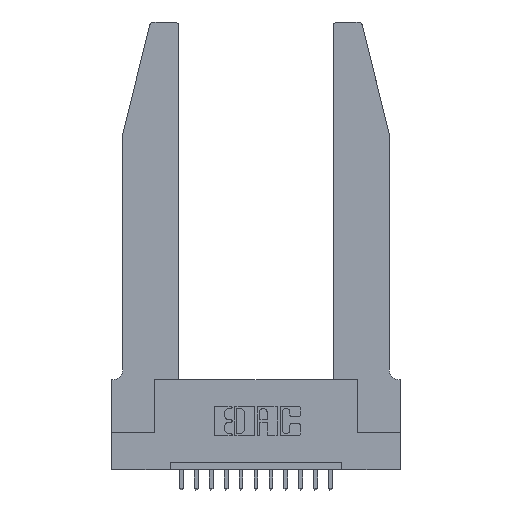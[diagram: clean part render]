
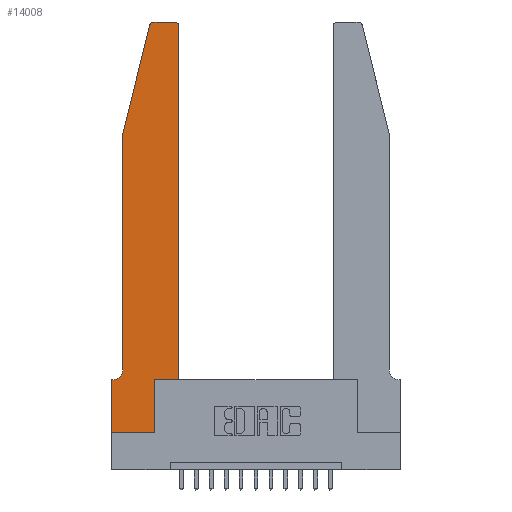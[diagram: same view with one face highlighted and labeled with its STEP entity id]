
A CAD part, top view. The second image highlights one B-rep face of the part: STEP entity #14008.
In plain terms, the highlighted planar face has unit normal (0, 0, 1).
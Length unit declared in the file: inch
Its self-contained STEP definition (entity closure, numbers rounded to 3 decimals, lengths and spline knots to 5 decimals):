
#631 = CARTESIAN_POINT ( 'NONE',  ( 0.284, 2.72, 0.37 ) ) ;
#816 = VECTOR ( 'NONE', #4452, 39.37008 ) ;
#818 = DIRECTION ( 'NONE',  ( -1., 0., 0. ) ) ;
#859 = CARTESIAN_POINT ( 'NONE',  ( 0.4205, 2.72, 0.37 ) ) ;
#905 = CARTESIAN_POINT ( 'NONE',  ( 0.0755, 2., 0.37 ) ) ;
#1058 = VERTEX_POINT ( 'NONE', #8115 ) ;
#1556 = CARTESIAN_POINT ( 'NONE',  ( 0., 0., 0.37 ) ) ;
#1710 = DIRECTION ( 'NONE',  ( 0., 1., 0. ) ) ;
#2097 = DIRECTION ( 'NONE',  ( 1., 0., 0. ) ) ;
#2115 = ORIENTED_EDGE ( 'NONE', *, *, #4178, .T. ) ;
#2126 = VERTEX_POINT ( 'NONE', #14077 ) ;
#2444 = VECTOR ( 'NONE', #7209, 39.37008 ) ;
#2479 = CARTESIAN_POINT ( 'NONE',  ( 0.0755, 2., 0.37 ) ) ;
#2604 = AXIS2_PLACEMENT_3D ( 'NONE', #859, #3654, #2097 ) ;
#2664 = ORIENTED_EDGE ( 'NONE', *, *, #14502, .T. ) ;
#2697 = DIRECTION ( 'NONE',  ( 1., 0., 0. ) ) ;
#2739 = LINE ( 'NONE', #905, #10667 ) ;
#2757 = EDGE_CURVE ( 'NONE', #12552, #12650, #2739, .T. ) ;
#2863 = EDGE_CURVE ( 'NONE', #2126, #11177, #6493, .T. ) ;
#3077 = AXIS2_PLACEMENT_3D ( 'NONE', #12010, #13465, #9400 ) ;
#3121 = CARTESIAN_POINT ( 'NONE',  ( 0.0055, 0.35, 0.37 ) ) ;
#3159 = EDGE_CURVE ( 'NONE', #8303, #13330, #5221, .T. ) ;
#3285 = VECTOR ( 'NONE', #2697, 39.37008 ) ;
#3375 = EDGE_LOOP ( 'NONE', ( #9673, #11715, #2115, #5408, #6092, #14903, #3936, #2664, #13091, #13509, #4253, #10044 ) ) ;
#3484 = VECTOR ( 'NONE', #14941, 39.37008 ) ;
#3654 = DIRECTION ( 'NONE',  ( 0., 0., 1. ) ) ;
#3880 = CIRCLE ( 'NONE', #15668, 0.03 ) ;
#3936 = ORIENTED_EDGE ( 'NONE', *, *, #11242, .T. ) ;
#4073 = VECTOR ( 'NONE', #11707, 39.37008 ) ;
#4130 = FACE_OUTER_BOUND ( 'NONE', #3375, .T. ) ;
#4178 = EDGE_CURVE ( 'NONE', #1058, #12552, #13865, .T. ) ;
#4253 = ORIENTED_EDGE ( 'NONE', *, *, #3159, .T. ) ;
#4269 = CARTESIAN_POINT ( 'NONE',  ( 0.2865, 0.35, 0.37 ) ) ;
#4452 = DIRECTION ( 'NONE',  ( -1., 0., 0. ) ) ;
#4743 = CARTESIAN_POINT ( 'NONE',  ( 0.4205, 2.75, 0.37 ) ) ;
#4809 = DIRECTION ( 'NONE',  ( 0., -1., 0. ) ) ;
#5166 = VECTOR ( 'NONE', #16021, 39.37008 ) ;
#5221 = LINE ( 'NONE', #14054, #11893 ) ;
#5408 = ORIENTED_EDGE ( 'NONE', *, *, #2757, .T. ) ;
#5464 = VERTEX_POINT ( 'NONE', #11940 ) ;
#5849 = EDGE_CURVE ( 'NONE', #12650, #13278, #13796, .T. ) ;
#6092 = ORIENTED_EDGE ( 'NONE', *, *, #5849, .T. ) ;
#6493 = LINE ( 'NONE', #16246, #13548 ) ;
#6675 = PLANE ( 'NONE',  #3077 ) ;
#6974 = CARTESIAN_POINT ( 'NONE',  ( 0.2605, 2.75, 0.37 ) ) ;
#7209 = DIRECTION ( 'NONE',  ( -1., 0., 0. ) ) ;
#7573 = CARTESIAN_POINT ( 'NONE',  ( 0.4505, 2.72, 0.37 ) ) ;
#8115 = CARTESIAN_POINT ( 'NONE',  ( 0.25487, 2.72718, 0.37 ) ) ;
#8129 = CARTESIAN_POINT ( 'NONE',  ( 0., 0., 0.37 ) ) ;
#8235 = CARTESIAN_POINT ( 'NONE',  ( 0.4505, 0.35, 0.37 ) ) ;
#8292 = CARTESIAN_POINT ( 'NONE',  ( 0.0755, 0.42, 0.37 ) ) ;
#8303 = VERTEX_POINT ( 'NONE', #14336 ) ;
#8323 = LINE ( 'NONE', #6974, #816 ) ;
#8956 = EDGE_CURVE ( 'NONE', #13853, #5464, #8323, .T. ) ;
#9400 = DIRECTION ( 'NONE',  ( 1., 0., 0. ) ) ;
#9673 = ORIENTED_EDGE ( 'NONE', *, *, #8956, .T. ) ;
#9903 = DIRECTION ( 'NONE',  ( 0., 0., 1. ) ) ;
#9987 = CARTESIAN_POINT ( 'NONE',  ( 0., 0.35, 0.37 ) ) ;
#10044 = ORIENTED_EDGE ( 'NONE', *, *, #11717, .T. ) ;
#10568 = LINE ( 'NONE', #1556, #3484 ) ;
#10667 = VECTOR ( 'NONE', #4809, 39.37008 ) ;
#11070 = EDGE_CURVE ( 'NONE', #5464, #1058, #3880, .T. ) ;
#11177 = VERTEX_POINT ( 'NONE', #4269 ) ;
#11242 = EDGE_CURVE ( 'NONE', #14239, #13611, #10568, .T. ) ;
#11426 = CARTESIAN_POINT ( 'NONE',  ( 0.0055, 0.42, 0.37 ) ) ;
#11427 = LINE ( 'NONE', #8129, #5166 ) ;
#11671 = EDGE_CURVE ( 'NONE', #13278, #14239, #12623, .T. ) ;
#11707 = DIRECTION ( 'NONE',  ( -0.239, -0.971, 0. ) ) ;
#11715 = ORIENTED_EDGE ( 'NONE', *, *, #11070, .T. ) ;
#11717 = EDGE_CURVE ( 'NONE', #13330, #13853, #14514, .T. ) ;
#11893 = VECTOR ( 'NONE', #15400, 39.37008 ) ;
#11940 = CARTESIAN_POINT ( 'NONE',  ( 0.284, 2.75, 0.37 ) ) ;
#12010 = CARTESIAN_POINT ( 'NONE',  ( 0., 0.35, 0.37 ) ) ;
#12341 = CARTESIAN_POINT ( 'NONE',  ( 0., 0., 0.37 ) ) ;
#12552 = VERTEX_POINT ( 'NONE', #2479 ) ;
#12623 = LINE ( 'NONE', #15180, #2444 ) ;
#12650 = VERTEX_POINT ( 'NONE', #8292 ) ;
#12685 = DIRECTION ( 'NONE',  ( 0., 0., -1. ) ) ;
#13080 = LINE ( 'NONE', #8235, #3285 ) ;
#13091 = ORIENTED_EDGE ( 'NONE', *, *, #2863, .T. ) ;
#13147 = CARTESIAN_POINT ( 'NONE',  ( 0.0755, 2., 0.37 ) ) ;
#13278 = VERTEX_POINT ( 'NONE', #3121 ) ;
#13330 = VERTEX_POINT ( 'NONE', #7573 ) ;
#13465 = DIRECTION ( 'NONE',  ( 0., 0., 1. ) ) ;
#13509 = ORIENTED_EDGE ( 'NONE', *, *, #14604, .T. ) ;
#13548 = VECTOR ( 'NONE', #1710, 39.37008 ) ;
#13611 = VERTEX_POINT ( 'NONE', #12341 ) ;
#13796 = CIRCLE ( 'NONE', #14716, 0.07 ) ;
#13853 = VERTEX_POINT ( 'NONE', #4743 ) ;
#13865 = LINE ( 'NONE', #13147, #4073 ) ;
#14008 = ADVANCED_FACE ( 'NONE', ( #4130 ), #6675, .T. ) ;
#14054 = CARTESIAN_POINT ( 'NONE',  ( 0.4505, 0.35, 0.37 ) ) ;
#14077 = CARTESIAN_POINT ( 'NONE',  ( 0.2865, 0., 0.37 ) ) ;
#14239 = VERTEX_POINT ( 'NONE', #9987 ) ;
#14336 = CARTESIAN_POINT ( 'NONE',  ( 0.4505, 0.35, 0.37 ) ) ;
#14502 = EDGE_CURVE ( 'NONE', #13611, #2126, #11427, .T. ) ;
#14514 = CIRCLE ( 'NONE', #2604, 0.03 ) ;
#14604 = EDGE_CURVE ( 'NONE', #11177, #8303, #13080, .T. ) ;
#14716 = AXIS2_PLACEMENT_3D ( 'NONE', #11426, #12685, #818 ) ;
#14903 = ORIENTED_EDGE ( 'NONE', *, *, #11671, .T. ) ;
#14941 = DIRECTION ( 'NONE',  ( 0., -1., 0. ) ) ;
#15180 = CARTESIAN_POINT ( 'NONE',  ( 0.0755, 0.35, 0.37 ) ) ;
#15400 = DIRECTION ( 'NONE',  ( 0., 1., 0. ) ) ;
#15668 = AXIS2_PLACEMENT_3D ( 'NONE', #631, #9903, #16583 ) ;
#16021 = DIRECTION ( 'NONE',  ( 1., 0., 0. ) ) ;
#16246 = CARTESIAN_POINT ( 'NONE',  ( 0.2865, 0.35, 0.37 ) ) ;
#16583 = DIRECTION ( 'NONE',  ( 1., 0., 0. ) ) ;
